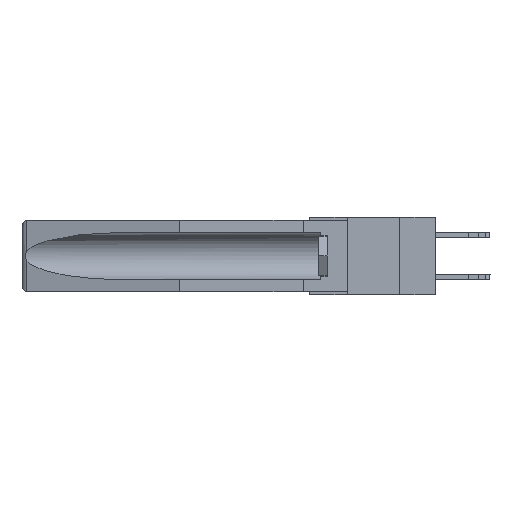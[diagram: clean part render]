
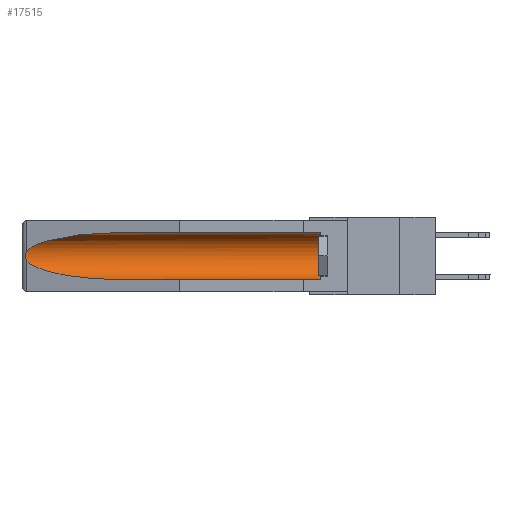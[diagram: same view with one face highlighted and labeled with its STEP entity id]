
A CAD part, left-side view. The second image highlights one B-rep face of the part: STEP entity #17515.
In plain terms, the highlighted cylindrical face has radius 2.857 mm (diameter 5.715 mm), a partial arc.
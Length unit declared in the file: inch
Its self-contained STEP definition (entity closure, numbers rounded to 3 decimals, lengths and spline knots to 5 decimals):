
#52 = CARTESIAN_POINT ( 'NONE',  ( 0.155, 0.126, -0.284 ) ) ;
#273 = VERTEX_POINT ( 'NONE', #52 ) ;
#669 = ORIENTED_EDGE ( 'NONE', *, *, #1484, .F. ) ;
#1031 = CARTESIAN_POINT ( 'NONE',  ( 0.26537, 1.52718, -0.14972 ) ) ;
#1484 = EDGE_CURVE ( 'NONE', #273, #24493, #23101, .T. ) ;
#1600 = CARTESIAN_POINT ( 'NONE',  ( 0.26537, 1.52718, -0.14972 ) ) ;
#1619 =( BOUNDED_CURVE ( )  B_SPLINE_CURVE ( 3, ( #14730, #12825, #4324, #8296 ),
 .UNSPECIFIED., .F., .F. ) 
 B_SPLINE_CURVE_WITH_KNOTS ( ( 4, 4 ),
 ( 4.71239, 6.08839 ),
 .UNSPECIFIED. ) 
 CURVE ( )  GEOMETRIC_REPRESENTATION_ITEM ( )  RATIONAL_B_SPLINE_CURVE ( ( 1., 0.848, 0.848, 1. ) ) 
 REPRESENTATION_ITEM ( '' )  );
#1685 = EDGE_CURVE ( 'NONE', #9884, #1874, #1619, .T. ) ;
#1826 = AXIS2_PLACEMENT_3D ( 'NONE', #14263, #18419, #18520 ) ;
#1874 = VERTEX_POINT ( 'NONE', #1600 ) ;
#2538 = ORIENTED_EDGE ( 'NONE', *, *, #21455, .T. ) ;
#3406 = DIRECTION ( 'NONE',  ( 0., 1., 0. ) ) ;
#3481 = CARTESIAN_POINT ( 'NONE',  ( 0.155, 0.126, -0.059 ) ) ;
#3536 = CARTESIAN_POINT ( 'NONE',  ( 0.26537, 1.52718, -0.19328 ) ) ;
#4324 = CARTESIAN_POINT ( 'NONE',  ( 0.25451, 1.48313, -0.09465 ) ) ;
#5160 = CARTESIAN_POINT ( 'NONE',  ( 0.26654, 1.53092, -0.15636 ) ) ;
#5229 = B_SPLINE_CURVE_WITH_KNOTS ( 'NONE', 3,
 ( #1031, #17554, #5160, #19646, #8297, #16350, #18438, #10398, #6308, #22577 ),
 .UNSPECIFIED., .F., .F.,
 ( 4, 2, 2, 2, 4 ),
 ( 0., 0.00029, 0.00058, 0.00087, 0.00117 ),
 .UNSPECIFIED. ) ;
#6308 = CARTESIAN_POINT ( 'NONE',  ( 0.26597, 1.5296, -0.19026 ) ) ;
#7786 = CARTESIAN_POINT ( 'NONE',  ( 0.21114, 1.30732, -0.284 ) ) ;
#7981 = EDGE_CURVE ( 'NONE', #10694, #24493, #18868, .T. ) ;
#8296 = CARTESIAN_POINT ( 'NONE',  ( 0.26537, 1.52718, -0.14972 ) ) ;
#8297 = CARTESIAN_POINT ( 'NONE',  ( 0.2675, 1.53308, -0.16763 ) ) ;
#9207 = CARTESIAN_POINT ( 'NONE',  ( 0.155, -0.30754, -0.059 ) ) ;
#9578 = VERTEX_POINT ( 'NONE', #3481 ) ;
#9657 = ORIENTED_EDGE ( 'NONE', *, *, #9725, .T. ) ;
#9725 = EDGE_CURVE ( 'NONE', #273, #9578, #25734, .T. ) ;
#9884 = VERTEX_POINT ( 'NONE', #20768 ) ;
#10398 = CARTESIAN_POINT ( 'NONE',  ( 0.26655, 1.53094, -0.18657 ) ) ;
#10694 = VERTEX_POINT ( 'NONE', #3536 ) ;
#11694 = LINE ( 'NONE', #9207, #23979 ) ;
#12323 = AXIS2_PLACEMENT_3D ( 'NONE', #17836, #18124, #26480 ) ;
#12825 = CARTESIAN_POINT ( 'NONE',  ( 0.21114, 1.30732, -0.059 ) ) ;
#12884 = EDGE_CURVE ( 'NONE', #9578, #9884, #11694, .T. ) ;
#13827 = DIRECTION ( 'NONE',  ( 0., 1., 0. ) ) ;
#13927 = CARTESIAN_POINT ( 'NONE',  ( 0.25451, 1.48313, -0.24835 ) ) ;
#14010 = CARTESIAN_POINT ( 'NONE',  ( 0.155, -0.30754, -0.284 ) ) ;
#14263 = CARTESIAN_POINT ( 'NONE',  ( 0.155, 0.126, -0.1715 ) ) ;
#14715 = CARTESIAN_POINT ( 'NONE',  ( 0.155, 1.07973, -0.284 ) ) ;
#14730 = CARTESIAN_POINT ( 'NONE',  ( 0.155, 1.07973, -0.059 ) ) ;
#16350 = CARTESIAN_POINT ( 'NONE',  ( 0.2675, 1.53308, -0.17534 ) ) ;
#16756 = ORIENTED_EDGE ( 'NONE', *, *, #1685, .T. ) ;
#17515 = ADVANCED_FACE ( 'NONE', ( #20200 ), #19233, .F. ) ;
#17554 = CARTESIAN_POINT ( 'NONE',  ( 0.26597, 1.52961, -0.15275 ) ) ;
#17836 = CARTESIAN_POINT ( 'NONE',  ( 0.155, -0.30754, -0.1715 ) ) ;
#18124 = DIRECTION ( 'NONE',  ( 0., 1., 0. ) ) ;
#18419 = DIRECTION ( 'NONE',  ( 0., -1., 0. ) ) ;
#18438 = CARTESIAN_POINT ( 'NONE',  ( 0.2673, 1.53269, -0.17917 ) ) ;
#18520 = DIRECTION ( 'NONE',  ( 0., 0., 1. ) ) ;
#18868 =( BOUNDED_CURVE ( )  B_SPLINE_CURVE ( 3, ( #26537, #13927, #7786, #24303 ),
 .UNSPECIFIED., .F., .F. ) 
 B_SPLINE_CURVE_WITH_KNOTS ( ( 4, 4 ),
 ( 0.1948, 1.5708 ),
 .UNSPECIFIED. ) 
 CURVE ( )  GEOMETRIC_REPRESENTATION_ITEM ( )  RATIONAL_B_SPLINE_CURVE ( ( 1., 0.848, 0.848, 1. ) ) 
 REPRESENTATION_ITEM ( '' )  );
#19233 = CYLINDRICAL_SURFACE ( 'NONE', #12323, 0.1125 ) ;
#19646 = CARTESIAN_POINT ( 'NONE',  ( 0.2673, 1.5327, -0.16383 ) ) ;
#20200 = FACE_OUTER_BOUND ( 'NONE', #25622, .T. ) ;
#20768 = CARTESIAN_POINT ( 'NONE',  ( 0.155, 1.07973, -0.059 ) ) ;
#21455 = EDGE_CURVE ( 'NONE', #1874, #10694, #5229, .T. ) ;
#22452 = VECTOR ( 'NONE', #3406, 39.37008 ) ;
#22577 = CARTESIAN_POINT ( 'NONE',  ( 0.26537, 1.52718, -0.19328 ) ) ;
#23101 = LINE ( 'NONE', #14010, #22452 ) ;
#23979 = VECTOR ( 'NONE', #13827, 39.37008 ) ;
#24303 = CARTESIAN_POINT ( 'NONE',  ( 0.155, 1.07973, -0.284 ) ) ;
#24493 = VERTEX_POINT ( 'NONE', #14715 ) ;
#24933 = ORIENTED_EDGE ( 'NONE', *, *, #12884, .T. ) ;
#25622 = EDGE_LOOP ( 'NONE', ( #16756, #2538, #26244, #669, #9657, #24933 ) ) ;
#25734 = CIRCLE ( 'NONE', #1826, 0.1125 ) ;
#26244 = ORIENTED_EDGE ( 'NONE', *, *, #7981, .T. ) ;
#26480 = DIRECTION ( 'NONE',  ( 0., 0., 1. ) ) ;
#26537 = CARTESIAN_POINT ( 'NONE',  ( 0.26537, 1.52718, -0.19328 ) ) ;
